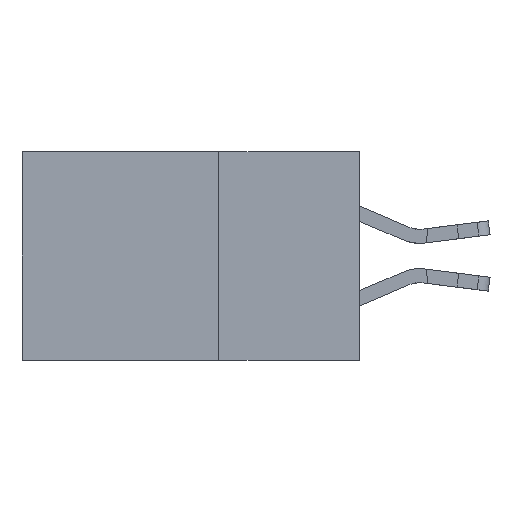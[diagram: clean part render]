
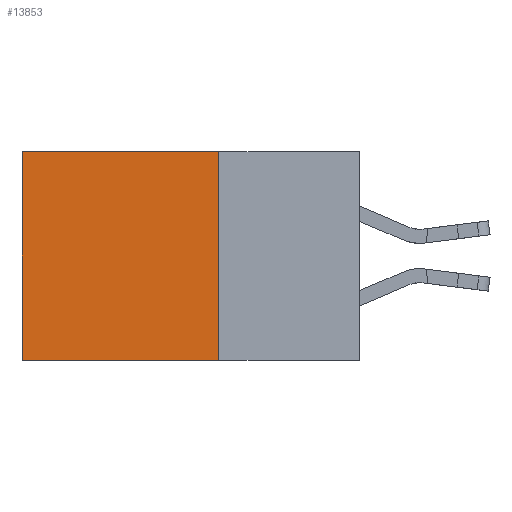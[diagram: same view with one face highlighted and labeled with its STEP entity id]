
A CAD part, left-side view. The second image highlights one B-rep face of the part: STEP entity #13853.
In plain terms, the highlighted planar face has unit normal (-1, 0, 0).
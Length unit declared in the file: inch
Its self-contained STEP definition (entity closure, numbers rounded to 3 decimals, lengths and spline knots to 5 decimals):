
#736 = LINE ( 'NONE', #26433, #21637 ) ;
#1272 = VECTOR ( 'NONE', #32455, 39.37008 ) ;
#2528 = DIRECTION ( 'NONE',  ( 0., 0., -1. ) ) ;
#2854 = EDGE_CURVE ( 'NONE', #14388, #24055, #15227, .T. ) ;
#3929 = CARTESIAN_POINT ( 'NONE',  ( 0.2875, 0.6, 0. ) ) ;
#4451 = ORIENTED_EDGE ( 'NONE', *, *, #2854, .T. ) ;
#5154 = LINE ( 'NONE', #17958, #11296 ) ;
#5459 = DIRECTION ( 'NONE',  ( 0., 0., -1. ) ) ;
#6343 = CARTESIAN_POINT ( 'NONE',  ( 0.2875, 0.6, -0.37 ) ) ;
#6733 = FACE_OUTER_BOUND ( 'NONE', #14943, .T. ) ;
#7930 = CARTESIAN_POINT ( 'NONE',  ( 0.2875, 0.25, 0. ) ) ;
#8716 = ORIENTED_EDGE ( 'NONE', *, *, #32464, .F. ) ;
#10029 = DIRECTION ( 'NONE',  ( 0., 0., -1. ) ) ;
#10552 = CARTESIAN_POINT ( 'NONE',  ( 0.2875, 0.25, -0.37 ) ) ;
#11296 = VECTOR ( 'NONE', #10029, 39.37008 ) ;
#12668 = VECTOR ( 'NONE', #28813, 39.37008 ) ;
#13853 = ADVANCED_FACE ( 'NONE', ( #6733 ), #15825, .F. ) ;
#14388 = VERTEX_POINT ( 'NONE', #7930 ) ;
#14943 = EDGE_LOOP ( 'NONE', ( #32895, #8716, #21469, #4451 ) ) ;
#15227 = LINE ( 'NONE', #21927, #1272 ) ;
#15825 = PLANE ( 'NONE',  #27020 ) ;
#17958 = CARTESIAN_POINT ( 'NONE',  ( 0.2875, 0.25, 0. ) ) ;
#19278 = EDGE_CURVE ( 'NONE', #24055, #29426, #736, .T. ) ;
#20778 = DIRECTION ( 'NONE',  ( 1., 0., 0. ) ) ;
#21469 = ORIENTED_EDGE ( 'NONE', *, *, #28940, .F. ) ;
#21637 = VECTOR ( 'NONE', #5459, 39.37008 ) ;
#21927 = CARTESIAN_POINT ( 'NONE',  ( 0.2875, 0.25, 0. ) ) ;
#24055 = VERTEX_POINT ( 'NONE', #3929 ) ;
#26233 = LINE ( 'NONE', #26383, #12668 ) ;
#26383 = CARTESIAN_POINT ( 'NONE',  ( 0.2875, 0.25, -0.37 ) ) ;
#26433 = CARTESIAN_POINT ( 'NONE',  ( 0.2875, 0.6, 0. ) ) ;
#27020 = AXIS2_PLACEMENT_3D ( 'NONE', #28677, #20778, #2528 ) ;
#28677 = CARTESIAN_POINT ( 'NONE',  ( 0.2875, 0.25, 0. ) ) ;
#28813 = DIRECTION ( 'NONE',  ( 0., 1., 0. ) ) ;
#28940 = EDGE_CURVE ( 'NONE', #14388, #32399, #5154, .T. ) ;
#29426 = VERTEX_POINT ( 'NONE', #6343 ) ;
#32399 = VERTEX_POINT ( 'NONE', #10552 ) ;
#32455 = DIRECTION ( 'NONE',  ( 0., 1., 0. ) ) ;
#32464 = EDGE_CURVE ( 'NONE', #32399, #29426, #26233, .T. ) ;
#32895 = ORIENTED_EDGE ( 'NONE', *, *, #19278, .T. ) ;
